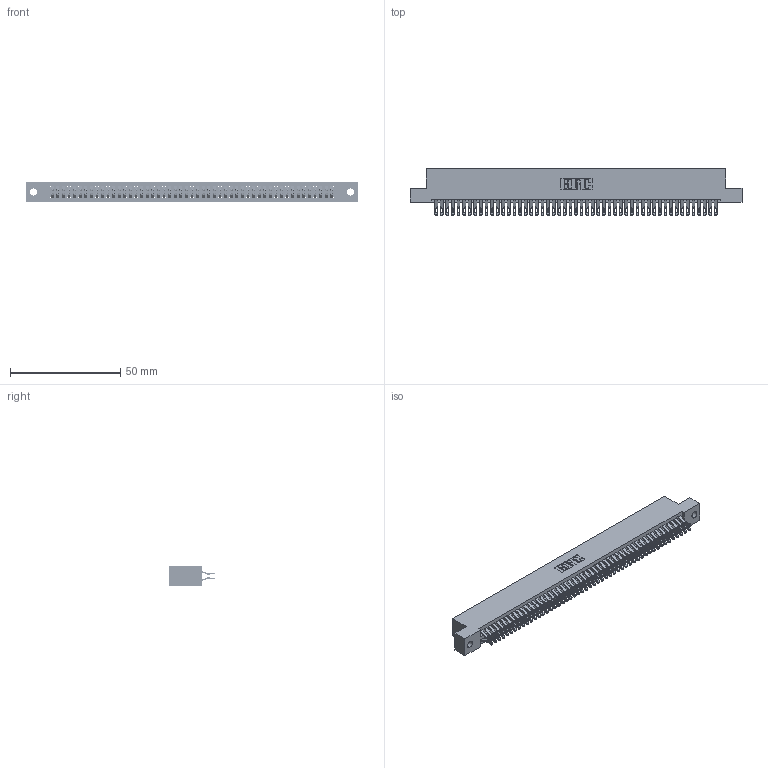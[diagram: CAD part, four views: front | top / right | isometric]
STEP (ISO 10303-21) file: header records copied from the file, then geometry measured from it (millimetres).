
FILE_DESCRIPTION (( 'STEP AP203' ), '1' );
FILE_NAME ('345-102-555-202.STEP', '2018-10-05T20:39:54', ( '' ), ( '' ), 'SwSTEP 2.0', 'SolidWorks 2016', '' );
FILE_SCHEMA (( 'CONFIG_CONTROL_DESIGN' ));
Length unit declared in the file: inch
Products named in the file (3): 345-102-555-202; 345-292-001_555 Tail; 345 Part_Flush Mounting Lugs - 0.128 Dia
Assembly tree (103 placements, depth 2):
  345-102-555-202
    345 Part_Flush Mounting Lugs - 0.128 Dia
    345-292-001_555 Tail  x102
Bounding box: 150.75 x 21.13 x 9.4 mm (x, y, z)
Volume: 14986.6 mm3; surface area: 23083.4 mm2
Topology: 103 solids, 103 shells, 5838 faces, 18395 edges, 12262 vertices
Faces by surface type: plane 3242, cylinder 2596
Entity records: 39133 total; most frequent: CARTESIAN_POINT 6586, ORIENTED_EDGE 6490, DIRECTION 5765, EDGE_CURVE 3245, VECTOR 2889, LINE 2889, VERTEX_POINT 2162, AXIS2_PLACEMENT_3D 1438
